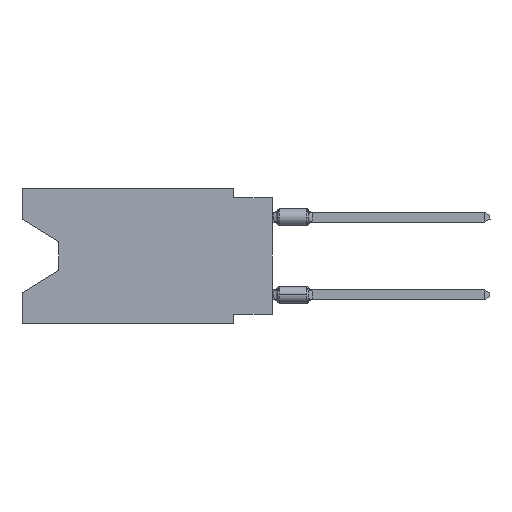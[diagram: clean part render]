
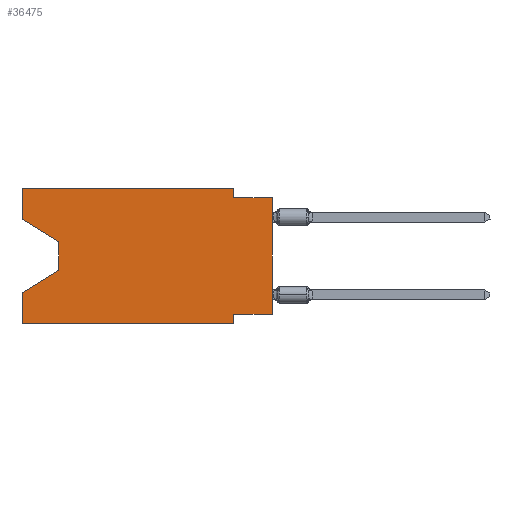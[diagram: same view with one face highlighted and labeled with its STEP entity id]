
A CAD part, left-side view. The second image highlights one B-rep face of the part: STEP entity #36475.
In plain terms, the highlighted planar face has unit normal (-1, 0, 0).
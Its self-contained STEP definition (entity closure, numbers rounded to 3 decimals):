
#727 = VECTOR ( 'NONE', #17745, 1000. ) ;
#963 = DIRECTION ( 'NONE',  ( 0., 0., 1. ) ) ;
#2229 = VECTOR ( 'NONE', #15430, 1000. ) ;
#2505 = EDGE_CURVE ( 'NONE', #18885, #15484, #16339, .T. ) ;
#3315 = LINE ( 'NONE', #7259, #25282 ) ;
#4004 = VECTOR ( 'NONE', #5486, 1000. ) ;
#5363 = DIRECTION ( 'NONE',  ( 0., -0.855, -0.519 ) ) ;
#5486 = DIRECTION ( 'NONE',  ( 0., 0., 1. ) ) ;
#6100 = DIRECTION ( 'NONE',  ( 0., 0., -1. ) ) ;
#6266 = VERTEX_POINT ( 'NONE', #49717 ) ;
#6987 = CARTESIAN_POINT ( 'NONE',  ( 0., 0., 0. ) ) ;
#7007 = DIRECTION ( 'NONE',  ( 1., 0., 0. ) ) ;
#7137 = EDGE_CURVE ( 'NONE', #28012, #18972, #46415, .T. ) ;
#7259 = CARTESIAN_POINT ( 'NONE',  ( 0., 16.383, 0. ) ) ;
#7530 = FACE_OUTER_BOUND ( 'NONE', #11341, .T. ) ;
#8202 = ORIENTED_EDGE ( 'NONE', *, *, #25962, .F. ) ;
#8264 = AXIS2_PLACEMENT_3D ( 'NONE', #51880, #7007, #43401 ) ;
#8325 = EDGE_CURVE ( 'NONE', #28012, #37367, #36115, .T. ) ;
#8692 = ORIENTED_EDGE ( 'NONE', *, *, #7137, .T. ) ;
#9635 = LINE ( 'NONE', #17270, #35158 ) ;
#10566 = DIRECTION ( 'NONE',  ( 0., 0., 1. ) ) ;
#10621 = CARTESIAN_POINT ( 'NONE',  ( 0., 16.383, -2.038 ) ) ;
#11341 = EDGE_LOOP ( 'NONE', ( #21031, #27051, #31903, #33788, #47021, #8202, #13705, #8692, #29373, #49913, #31484, #33491 ) ) ;
#12551 = VECTOR ( 'NONE', #10566, 1000. ) ;
#13101 = VERTEX_POINT ( 'NONE', #16311 ) ;
#13705 = ORIENTED_EDGE ( 'NONE', *, *, #8325, .F. ) ;
#13875 = CARTESIAN_POINT ( 'NONE',  ( 0., 13.97, -3.505 ) ) ;
#14035 = CARTESIAN_POINT ( 'NONE',  ( 0., 2.54, -0.635 ) ) ;
#14478 = CARTESIAN_POINT ( 'NONE',  ( 0., 2.54, 0. ) ) ;
#14875 = EDGE_CURVE ( 'NONE', #6266, #13101, #9635, .T. ) ;
#15070 = VECTOR ( 'NONE', #5363, 1000. ) ;
#15341 = VERTEX_POINT ( 'NONE', #48935 ) ;
#15430 = DIRECTION ( 'NONE',  ( 0., 0.855, -0.519 ) ) ;
#15484 = VERTEX_POINT ( 'NONE', #14035 ) ;
#16311 = CARTESIAN_POINT ( 'NONE',  ( 0., 16.383, 0. ) ) ;
#16339 = LINE ( 'NONE', #35872, #41103 ) ;
#17270 = CARTESIAN_POINT ( 'NONE',  ( 0., 16.383, 0. ) ) ;
#17696 = VECTOR ( 'NONE', #29980, 1000. ) ;
#17745 = DIRECTION ( 'NONE',  ( 0., -1., 0. ) ) ;
#17970 = LINE ( 'NONE', #34327, #21795 ) ;
#18885 = VERTEX_POINT ( 'NONE', #14478 ) ;
#18945 = VERTEX_POINT ( 'NONE', #27388 ) ;
#18972 = VERTEX_POINT ( 'NONE', #44262 ) ;
#20308 = DIRECTION ( 'NONE',  ( 0., 0., -1. ) ) ;
#20823 = VECTOR ( 'NONE', #21056, 1000. ) ;
#21031 = ORIENTED_EDGE ( 'NONE', *, *, #24329, .T. ) ;
#21056 = DIRECTION ( 'NONE',  ( 0., -1., 0. ) ) ;
#21795 = VECTOR ( 'NONE', #6100, 1000. ) ;
#22181 = CARTESIAN_POINT ( 'NONE',  ( 0., 16.383, 0. ) ) ;
#22986 = VERTEX_POINT ( 'NONE', #40445 ) ;
#24329 = EDGE_CURVE ( 'NONE', #6266, #18945, #41751, .T. ) ;
#25282 = VECTOR ( 'NONE', #43408, 1000. ) ;
#25962 = EDGE_CURVE ( 'NONE', #37367, #33305, #17970, .T. ) ;
#25995 = EDGE_CURVE ( 'NONE', #22986, #28072, #46487, .T. ) ;
#27051 = ORIENTED_EDGE ( 'NONE', *, *, #40436, .T. ) ;
#27388 = CARTESIAN_POINT ( 'NONE',  ( 0., 13.97, -3.505 ) ) ;
#27937 = DIRECTION ( 'NONE',  ( 0., 1., 0. ) ) ;
#28012 = VERTEX_POINT ( 'NONE', #33669 ) ;
#28072 = VERTEX_POINT ( 'NONE', #41568 ) ;
#29373 = ORIENTED_EDGE ( 'NONE', *, *, #47046, .F. ) ;
#29980 = DIRECTION ( 'NONE',  ( 0., 0., -1. ) ) ;
#31067 = VECTOR ( 'NONE', #27937, 1000. ) ;
#31484 = ORIENTED_EDGE ( 'NONE', *, *, #40505, .F. ) ;
#31797 = CARTESIAN_POINT ( 'NONE',  ( 0., 13.97, -5.385 ) ) ;
#31903 = ORIENTED_EDGE ( 'NONE', *, *, #34834, .T. ) ;
#33305 = VERTEX_POINT ( 'NONE', #49448 ) ;
#33491 = ORIENTED_EDGE ( 'NONE', *, *, #14875, .F. ) ;
#33669 = CARTESIAN_POINT ( 'NONE',  ( 0., 0., -8.255 ) ) ;
#33788 = ORIENTED_EDGE ( 'NONE', *, *, #25995, .F. ) ;
#34327 = CARTESIAN_POINT ( 'NONE',  ( 0., 2.54, -8.89 ) ) ;
#34834 = EDGE_CURVE ( 'NONE', #15341, #28072, #35223, .T. ) ;
#35158 = VECTOR ( 'NONE', #963, 1000. ) ;
#35223 = LINE ( 'NONE', #31797, #2229 ) ;
#35872 = CARTESIAN_POINT ( 'NONE',  ( 0., 2.54, 0. ) ) ;
#36115 = LINE ( 'NONE', #48275, #31067 ) ;
#36475 = ADVANCED_FACE ( 'NONE', ( #7530 ), #51348, .F. ) ;
#37367 = VERTEX_POINT ( 'NONE', #50954 ) ;
#40436 = EDGE_CURVE ( 'NONE', #18945, #15341, #50063, .T. ) ;
#40445 = CARTESIAN_POINT ( 'NONE',  ( 0., 16.383, -8.89 ) ) ;
#40505 = EDGE_CURVE ( 'NONE', #13101, #18885, #3315, .T. ) ;
#41103 = VECTOR ( 'NONE', #20308, 1000. ) ;
#41568 = CARTESIAN_POINT ( 'NONE',  ( 0., 16.383, -6.852 ) ) ;
#41732 = CARTESIAN_POINT ( 'NONE',  ( 0., 16.383, -8.89 ) ) ;
#41751 = LINE ( 'NONE', #10621, #15070 ) ;
#43401 = DIRECTION ( 'NONE',  ( 0., 0., -1. ) ) ;
#43408 = DIRECTION ( 'NONE',  ( 0., -1., 0. ) ) ;
#44262 = CARTESIAN_POINT ( 'NONE',  ( 0., 0., -0.635 ) ) ;
#44294 = LINE ( 'NONE', #45076, #20823 ) ;
#45076 = CARTESIAN_POINT ( 'NONE',  ( 0., 0., -0.635 ) ) ;
#46415 = LINE ( 'NONE', #6987, #4004 ) ;
#46487 = LINE ( 'NONE', #22181, #12551 ) ;
#47021 = ORIENTED_EDGE ( 'NONE', *, *, #50514, .T. ) ;
#47046 = EDGE_CURVE ( 'NONE', #15484, #18972, #44294, .T. ) ;
#48275 = CARTESIAN_POINT ( 'NONE',  ( 0., 0., -8.255 ) ) ;
#48935 = CARTESIAN_POINT ( 'NONE',  ( 0., 13.97, -5.385 ) ) ;
#49448 = CARTESIAN_POINT ( 'NONE',  ( 0., 2.54, -8.89 ) ) ;
#49717 = CARTESIAN_POINT ( 'NONE',  ( 0., 16.383, -2.038 ) ) ;
#49913 = ORIENTED_EDGE ( 'NONE', *, *, #2505, .F. ) ;
#49969 = LINE ( 'NONE', #41732, #727 ) ;
#50063 = LINE ( 'NONE', #13875, #17696 ) ;
#50514 = EDGE_CURVE ( 'NONE', #22986, #33305, #49969, .T. ) ;
#50954 = CARTESIAN_POINT ( 'NONE',  ( 0., 2.54, -8.255 ) ) ;
#51348 = PLANE ( 'NONE',  #8264 ) ;
#51880 = CARTESIAN_POINT ( 'NONE',  ( 0., 16.383, 0. ) ) ;
